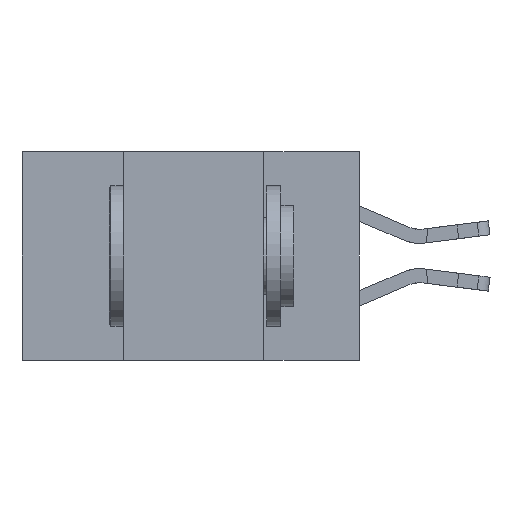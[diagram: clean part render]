
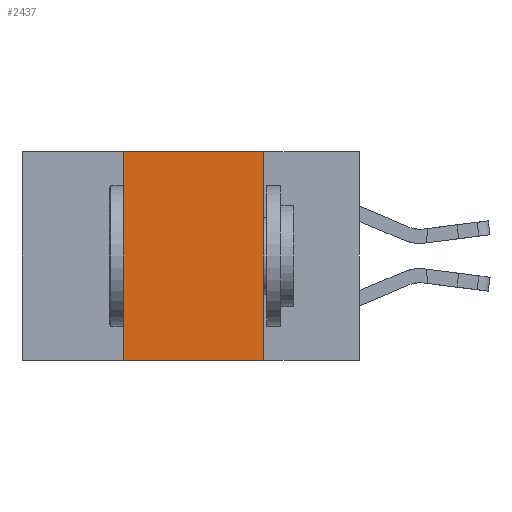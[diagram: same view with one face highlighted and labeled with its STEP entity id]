
A CAD part, left-side view. The second image highlights one B-rep face of the part: STEP entity #2437.
In plain terms, the highlighted planar face has unit normal (-1, 0, 0).
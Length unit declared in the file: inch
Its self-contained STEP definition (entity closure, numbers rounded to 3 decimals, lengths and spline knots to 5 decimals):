
#1129 = ORIENTED_EDGE ( 'NONE', *, *, #16505, .F. ) ;
#1190 = EDGE_LOOP ( 'NONE', ( #3189, #14599, #1129, #1312 ) ) ;
#1269 = DIRECTION ( 'NONE',  ( 1., 0., 0. ) ) ;
#1312 = ORIENTED_EDGE ( 'NONE', *, *, #14132, .T. ) ;
#1441 = CARTESIAN_POINT ( 'NONE',  ( 0., 0.6, -0.37 ) ) ;
#2437 = ADVANCED_FACE ( 'NONE', ( #10080 ), #4060, .F. ) ;
#2919 = CARTESIAN_POINT ( 'NONE',  ( 0., 0.17, -0.37 ) ) ;
#3145 = CARTESIAN_POINT ( 'NONE',  ( 0., 0.42, 0. ) ) ;
#3189 = ORIENTED_EDGE ( 'NONE', *, *, #15706, .F. ) ;
#4060 = PLANE ( 'NONE',  #9017 ) ;
#4444 = VERTEX_POINT ( 'NONE', #6608 ) ;
#5065 = VECTOR ( 'NONE', #14152, 39.37008 ) ;
#5129 = CARTESIAN_POINT ( 'NONE',  ( 0., 0.42, 0. ) ) ;
#5949 = CARTESIAN_POINT ( 'NONE',  ( 0., 0.42, -0.37 ) ) ;
#6608 = CARTESIAN_POINT ( 'NONE',  ( 0., 0.17, 0. ) ) ;
#7851 = VERTEX_POINT ( 'NONE', #3145 ) ;
#7860 = DIRECTION ( 'NONE',  ( 0., 0., 1. ) ) ;
#8448 = LINE ( 'NONE', #1441, #5065 ) ;
#9017 = AXIS2_PLACEMENT_3D ( 'NONE', #11483, #1269, #11603 ) ;
#9084 = DIRECTION ( 'NONE',  ( 0., -1., 0. ) ) ;
#10004 = VERTEX_POINT ( 'NONE', #2919 ) ;
#10080 = FACE_OUTER_BOUND ( 'NONE', #1190, .T. ) ;
#10227 = LINE ( 'NONE', #16072, #11819 ) ;
#11483 = CARTESIAN_POINT ( 'NONE',  ( 0., 0.6, 0. ) ) ;
#11589 = VERTEX_POINT ( 'NONE', #5949 ) ;
#11603 = DIRECTION ( 'NONE',  ( 0., 0., -1. ) ) ;
#11628 = VECTOR ( 'NONE', #9084, 39.37008 ) ;
#11819 = VECTOR ( 'NONE', #12128, 39.37008 ) ;
#12019 = LINE ( 'NONE', #12823, #11628 ) ;
#12128 = DIRECTION ( 'NONE',  ( 0., 0., -1. ) ) ;
#12823 = CARTESIAN_POINT ( 'NONE',  ( 0., 0.6, 0. ) ) ;
#13843 = EDGE_CURVE ( 'NONE', #7851, #4444, #12019, .T. ) ;
#14132 = EDGE_CURVE ( 'NONE', #11589, #10004, #8448, .T. ) ;
#14152 = DIRECTION ( 'NONE',  ( 0., -1., 0. ) ) ;
#14599 = ORIENTED_EDGE ( 'NONE', *, *, #13843, .F. ) ;
#14816 = LINE ( 'NONE', #5129, #15826 ) ;
#15706 = EDGE_CURVE ( 'NONE', #4444, #10004, #10227, .T. ) ;
#15826 = VECTOR ( 'NONE', #7860, 39.37008 ) ;
#16072 = CARTESIAN_POINT ( 'NONE',  ( 0., 0.17, 0. ) ) ;
#16505 = EDGE_CURVE ( 'NONE', #11589, #7851, #14816, .T. ) ;
